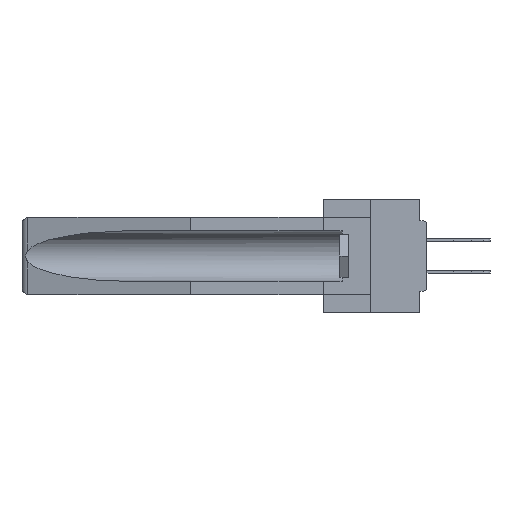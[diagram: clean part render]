
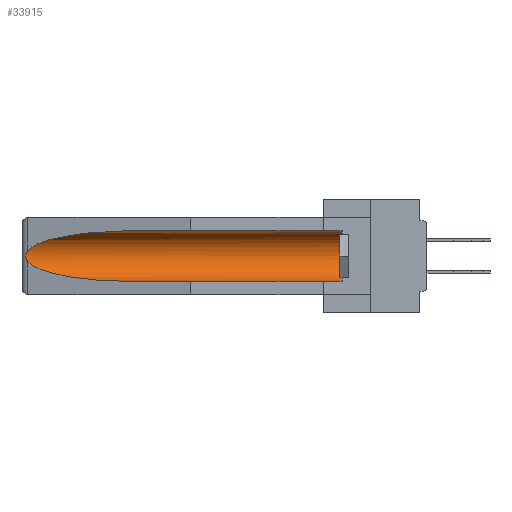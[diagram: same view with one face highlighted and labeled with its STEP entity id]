
A CAD part, left-side view. The second image highlights one B-rep face of the part: STEP entity #33915.
In plain terms, the highlighted cylindrical face has radius 2.857 mm (diameter 5.715 mm), a partial arc.
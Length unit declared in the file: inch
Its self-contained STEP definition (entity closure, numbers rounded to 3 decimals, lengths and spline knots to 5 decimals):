
#666 = CARTESIAN_POINT ( 'NONE',  ( 0.26597, 1.52961, -0.15275 ) ) ;
#3133 = CARTESIAN_POINT ( 'NONE',  ( 0.155, 1.07973, -0.284 ) ) ;
#3255 = CARTESIAN_POINT ( 'NONE',  ( 0.155, -0.30754, -0.1715 ) ) ;
#3601 = CARTESIAN_POINT ( 'NONE',  ( 0.25451, 1.48313, -0.24835 ) ) ;
#5017 = CARTESIAN_POINT ( 'NONE',  ( 0.26537, 1.52718, -0.14972 ) ) ;
#6405 = CIRCLE ( 'NONE', #13649, 0.1125 ) ;
#8168 = DIRECTION ( 'NONE',  ( 0., 1., 0. ) ) ;
#10073 = VECTOR ( 'NONE', #8168, 39.37008 ) ;
#10231 = VERTEX_POINT ( 'NONE', #39516 ) ;
#10678 = LINE ( 'NONE', #37467, #10073 ) ;
#12004 = CARTESIAN_POINT ( 'NONE',  ( 0.155, 1.07973, -0.059 ) ) ;
#13314 = CARTESIAN_POINT ( 'NONE',  ( 0.155, -0.30754, -0.284 ) ) ;
#13358 = AXIS2_PLACEMENT_3D ( 'NONE', #3255, #39856, #35862 ) ;
#13649 = AXIS2_PLACEMENT_3D ( 'NONE', #14302, #46765, #25580 ) ;
#14302 = CARTESIAN_POINT ( 'NONE',  ( 0.155, 0.126, -0.1715 ) ) ;
#15256 = CARTESIAN_POINT ( 'NONE',  ( 0.26597, 1.5296, -0.19026 ) ) ;
#15882 =( BOUNDED_CURVE ( )  B_SPLINE_CURVE ( 3, ( #17563, #3601, #36060, #3133 ),
 .UNSPECIFIED., .F., .F. ) 
 B_SPLINE_CURVE_WITH_KNOTS ( ( 4, 4 ),
 ( 0.1948, 1.5708 ),
 .UNSPECIFIED. ) 
 CURVE ( )  GEOMETRIC_REPRESENTATION_ITEM ( )  RATIONAL_B_SPLINE_CURVE ( ( 1., 0.848, 0.848, 1. ) ) 
 REPRESENTATION_ITEM ( '' )  );
#16453 = ORIENTED_EDGE ( 'NONE', *, *, #38893, .T. ) ;
#17563 = CARTESIAN_POINT ( 'NONE',  ( 0.26537, 1.52718, -0.19328 ) ) ;
#17686 = ORIENTED_EDGE ( 'NONE', *, *, #18758, .T. ) ;
#18173 = EDGE_CURVE ( 'NONE', #43101, #10231, #32072, .T. ) ;
#18751 = CARTESIAN_POINT ( 'NONE',  ( 0.26654, 1.53092, -0.15636 ) ) ;
#18758 = EDGE_CURVE ( 'NONE', #44483, #43101, #18836, .T. ) ;
#18836 =( BOUNDED_CURVE ( )  B_SPLINE_CURVE ( 3, ( #12004, #30191, #37510, #5017 ),
 .UNSPECIFIED., .F., .T. ) 
 B_SPLINE_CURVE_WITH_KNOTS ( ( 4, 4 ),
 ( 4.71239, 6.08839 ),
 .UNSPECIFIED. ) 
 CURVE ( )  GEOMETRIC_REPRESENTATION_ITEM ( )  RATIONAL_B_SPLINE_CURVE ( ( 1., 0.848, 0.848, 1. ) ) 
 REPRESENTATION_ITEM ( '' )  );
#19432 = EDGE_LOOP ( 'NONE', ( #17686, #44257, #16453, #36924, #45967, #39525 ) ) ;
#22325 = EDGE_CURVE ( 'NONE', #39415, #32681, #6405, .T. ) ;
#24383 = EDGE_CURVE ( 'NONE', #39415, #36421, #44247, .T. ) ;
#25580 = DIRECTION ( 'NONE',  ( 0., 0., 1. ) ) ;
#28357 = CARTESIAN_POINT ( 'NONE',  ( 0.26537, 1.52718, -0.14972 ) ) ;
#30191 = CARTESIAN_POINT ( 'NONE',  ( 0.21114, 1.30732, -0.059 ) ) ;
#30639 = VECTOR ( 'NONE', #35464, 39.37008 ) ;
#31358 = CARTESIAN_POINT ( 'NONE',  ( 0.155, 0.126, -0.059 ) ) ;
#31449 = CARTESIAN_POINT ( 'NONE',  ( 0.155, 1.07973, -0.284 ) ) ;
#32014 = FACE_OUTER_BOUND ( 'NONE', #19432, .T. ) ;
#32072 = B_SPLINE_CURVE_WITH_KNOTS ( 'NONE', 3,
 ( #40415, #666, #18751, #40100, #44043, #43886, #36449, #36930, #15256, #40567 ),
 .UNSPECIFIED., .F., .F.,
 ( 4, 2, 2, 2, 4 ),
 ( 0., 0.00029, 0.00058, 0.00087, 0.00117 ),
 .UNSPECIFIED. ) ;
#32681 = VERTEX_POINT ( 'NONE', #31358 ) ;
#33106 = EDGE_CURVE ( 'NONE', #32681, #44483, #10678, .T. ) ;
#33915 = ADVANCED_FACE ( 'NONE', ( #32014 ), #42830, .F. ) ;
#33950 = CARTESIAN_POINT ( 'NONE',  ( 0.155, 1.07973, -0.059 ) ) ;
#35464 = DIRECTION ( 'NONE',  ( 0., 1., 0. ) ) ;
#35862 = DIRECTION ( 'NONE',  ( 0., 0., 1. ) ) ;
#36060 = CARTESIAN_POINT ( 'NONE',  ( 0.21114, 1.30732, -0.284 ) ) ;
#36421 = VERTEX_POINT ( 'NONE', #31449 ) ;
#36449 = CARTESIAN_POINT ( 'NONE',  ( 0.2673, 1.53269, -0.17917 ) ) ;
#36924 = ORIENTED_EDGE ( 'NONE', *, *, #24383, .F. ) ;
#36930 = CARTESIAN_POINT ( 'NONE',  ( 0.26655, 1.53094, -0.18657 ) ) ;
#37467 = CARTESIAN_POINT ( 'NONE',  ( 0.155, -0.30754, -0.059 ) ) ;
#37510 = CARTESIAN_POINT ( 'NONE',  ( 0.25451, 1.48313, -0.09465 ) ) ;
#38893 = EDGE_CURVE ( 'NONE', #10231, #36421, #15882, .T. ) ;
#39415 = VERTEX_POINT ( 'NONE', #39940 ) ;
#39516 = CARTESIAN_POINT ( 'NONE',  ( 0.26537, 1.52718, -0.19328 ) ) ;
#39525 = ORIENTED_EDGE ( 'NONE', *, *, #33106, .T. ) ;
#39856 = DIRECTION ( 'NONE',  ( 0., 1., 0. ) ) ;
#39940 = CARTESIAN_POINT ( 'NONE',  ( 0.155, 0.126, -0.284 ) ) ;
#40100 = CARTESIAN_POINT ( 'NONE',  ( 0.2673, 1.5327, -0.16383 ) ) ;
#40415 = CARTESIAN_POINT ( 'NONE',  ( 0.26537, 1.52718, -0.14972 ) ) ;
#40567 = CARTESIAN_POINT ( 'NONE',  ( 0.26537, 1.52718, -0.19328 ) ) ;
#42830 = CYLINDRICAL_SURFACE ( 'NONE', #13358, 0.1125 ) ;
#43101 = VERTEX_POINT ( 'NONE', #28357 ) ;
#43886 = CARTESIAN_POINT ( 'NONE',  ( 0.2675, 1.53308, -0.17534 ) ) ;
#44043 = CARTESIAN_POINT ( 'NONE',  ( 0.2675, 1.53308, -0.16763 ) ) ;
#44247 = LINE ( 'NONE', #13314, #30639 ) ;
#44257 = ORIENTED_EDGE ( 'NONE', *, *, #18173, .T. ) ;
#44483 = VERTEX_POINT ( 'NONE', #33950 ) ;
#45967 = ORIENTED_EDGE ( 'NONE', *, *, #22325, .T. ) ;
#46765 = DIRECTION ( 'NONE',  ( 0., -1., 0. ) ) ;
